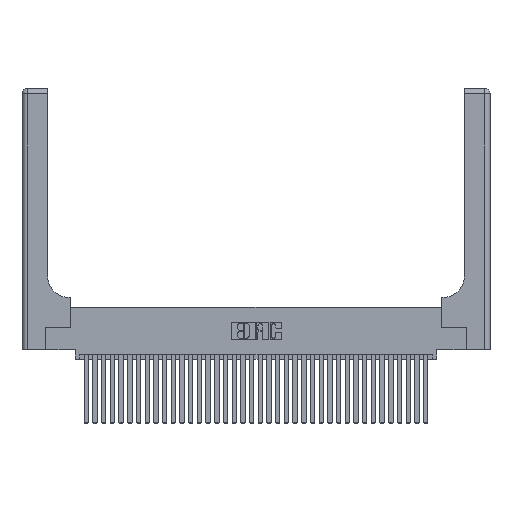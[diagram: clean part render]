
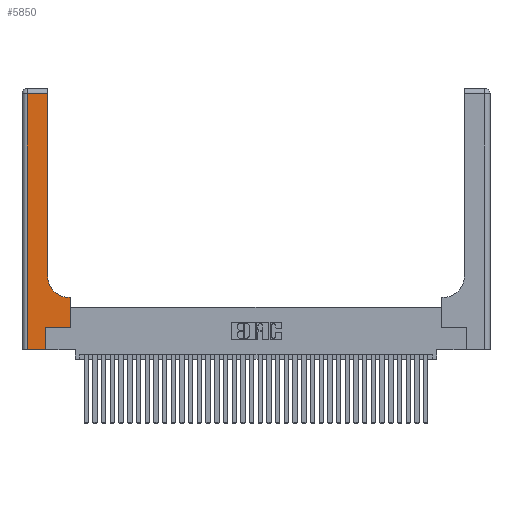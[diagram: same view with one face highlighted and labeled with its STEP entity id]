
A CAD part, top view. The second image highlights one B-rep face of the part: STEP entity #5850.
In plain terms, the highlighted planar face has unit normal (0, 0, 1).
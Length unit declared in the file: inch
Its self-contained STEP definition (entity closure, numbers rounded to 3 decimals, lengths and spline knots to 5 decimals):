
#67 = CARTESIAN_POINT ( 'NONE',  ( 0.5585, 0.25, 0.37 ) ) ;
#528 = CARTESIAN_POINT ( 'NONE',  ( 0.5585, 0.25, 0.37 ) ) ;
#1743 = LINE ( 'NONE', #5448, #31032 ) ;
#1891 = AXIS2_PLACEMENT_3D ( 'NONE', #32146, #15350, #34971 ) ;
#2219 = LINE ( 'NONE', #528, #16575 ) ;
#2608 = ORIENTED_EDGE ( 'NONE', *, *, #20187, .T. ) ;
#3395 = CARTESIAN_POINT ( 'NONE',  ( 0.5585, 0.6, 0.37 ) ) ;
#4171 = VERTEX_POINT ( 'NONE', #67 ) ;
#4239 = VERTEX_POINT ( 'NONE', #3395 ) ;
#5036 = CIRCLE ( 'NONE', #1891, 0.25 ) ;
#5448 = CARTESIAN_POINT ( 'NONE',  ( 0.06, 3., 0.37 ) ) ;
#5617 = EDGE_CURVE ( 'NONE', #33675, #6988, #1743, .T. ) ;
#5850 = ADVANCED_FACE ( 'NONE', ( #25758 ), #29022, .F. ) ;
#6583 = VECTOR ( 'NONE', #8959, 39.37008 ) ;
#6988 = VERTEX_POINT ( 'NONE', #28224 ) ;
#7287 = DIRECTION ( 'NONE',  ( 1., 0., 0. ) ) ;
#8959 = DIRECTION ( 'NONE',  ( 1., 0., 0. ) ) ;
#9021 = DIRECTION ( 'NONE',  ( -1., 0., 0. ) ) ;
#9207 = EDGE_CURVE ( 'NONE', #4239, #23665, #20814, .T. ) ;
#10063 = CARTESIAN_POINT ( 'NONE',  ( 0.2915, 2.94, 0.37 ) ) ;
#11771 = LINE ( 'NONE', #27359, #25807 ) ;
#12192 = AXIS2_PLACEMENT_3D ( 'NONE', #12219, #15021, #34631 ) ;
#12219 = CARTESIAN_POINT ( 'NONE',  ( 0., 3., 0.37 ) ) ;
#13022 = EDGE_CURVE ( 'NONE', #4171, #4239, #2219, .T. ) ;
#13323 = ORIENTED_EDGE ( 'NONE', *, *, #13022, .T. ) ;
#13383 = DIRECTION ( 'NONE',  ( -1., 0., 0. ) ) ;
#14323 = DIRECTION ( 'NONE',  ( 0., 1., 0. ) ) ;
#15021 = DIRECTION ( 'NONE',  ( 0., 0., -1. ) ) ;
#15350 = DIRECTION ( 'NONE',  ( 0., 0., -1. ) ) ;
#16575 = VECTOR ( 'NONE', #17768, 39.37008 ) ;
#17206 = EDGE_CURVE ( 'NONE', #22782, #24727, #25073, .T. ) ;
#17446 = VERTEX_POINT ( 'NONE', #35162 ) ;
#17768 = DIRECTION ( 'NONE',  ( 0., 1., 0. ) ) ;
#17877 = CARTESIAN_POINT ( 'NONE',  ( 0.2915, 0.6, 0.37 ) ) ;
#18522 = CARTESIAN_POINT ( 'NONE',  ( 0.2915, 0.85, 0.37 ) ) ;
#18593 = ORIENTED_EDGE ( 'NONE', *, *, #5617, .T. ) ;
#18896 = EDGE_CURVE ( 'NONE', #24727, #33675, #11771, .T. ) ;
#20073 = ORIENTED_EDGE ( 'NONE', *, *, #18896, .T. ) ;
#20187 = EDGE_CURVE ( 'NONE', #23665, #22782, #5036, .T. ) ;
#20488 = ORIENTED_EDGE ( 'NONE', *, *, #24462, .T. ) ;
#20814 = LINE ( 'NONE', #17877, #28295 ) ;
#21274 = LINE ( 'NONE', #22793, #34390 ) ;
#22116 = DIRECTION ( 'NONE',  ( 0., 1., 0. ) ) ;
#22427 = DIRECTION ( 'NONE',  ( 0., -1., 0. ) ) ;
#22503 = LINE ( 'NONE', #25791, #6583 ) ;
#22567 = VECTOR ( 'NONE', #7287, 39.37008 ) ;
#22782 = VERTEX_POINT ( 'NONE', #18522 ) ;
#22793 = CARTESIAN_POINT ( 'NONE',  ( 0.269, 0., 0.37 ) ) ;
#22799 = EDGE_CURVE ( 'NONE', #33431, #4171, #30030, .T. ) ;
#22839 = EDGE_LOOP ( 'NONE', ( #34150, #20073, #18593, #20488, #26024, #29378, #13323, #36374, #2608 ) ) ;
#23665 = VERTEX_POINT ( 'NONE', #24008 ) ;
#24008 = CARTESIAN_POINT ( 'NONE',  ( 0.5415, 0.6, 0.37 ) ) ;
#24462 = EDGE_CURVE ( 'NONE', #6988, #17446, #22503, .T. ) ;
#24727 = VERTEX_POINT ( 'NONE', #10063 ) ;
#24925 = CARTESIAN_POINT ( 'NONE',  ( 0.2915, 3., 0.37 ) ) ;
#25073 = LINE ( 'NONE', #24925, #30773 ) ;
#25758 = FACE_OUTER_BOUND ( 'NONE', #22839, .T. ) ;
#25791 = CARTESIAN_POINT ( 'NONE',  ( 0., 0., 0.37 ) ) ;
#25807 = VECTOR ( 'NONE', #13383, 39.37008 ) ;
#26024 = ORIENTED_EDGE ( 'NONE', *, *, #34575, .T. ) ;
#26289 = CARTESIAN_POINT ( 'NONE',  ( 0.269, 0.25, 0.37 ) ) ;
#27359 = CARTESIAN_POINT ( 'NONE',  ( 0., 2.94, 0.37 ) ) ;
#28224 = CARTESIAN_POINT ( 'NONE',  ( 0.06, 0., 0.37 ) ) ;
#28295 = VECTOR ( 'NONE', #9021, 39.37008 ) ;
#29022 = PLANE ( 'NONE',  #12192 ) ;
#29378 = ORIENTED_EDGE ( 'NONE', *, *, #22799, .T. ) ;
#29974 = CARTESIAN_POINT ( 'NONE',  ( 0.06, 2.94, 0.37 ) ) ;
#30030 = LINE ( 'NONE', #35313, #22567 ) ;
#30773 = VECTOR ( 'NONE', #22116, 39.37008 ) ;
#31032 = VECTOR ( 'NONE', #22427, 39.37008 ) ;
#32146 = CARTESIAN_POINT ( 'NONE',  ( 0.5415, 0.85, 0.37 ) ) ;
#33431 = VERTEX_POINT ( 'NONE', #26289 ) ;
#33675 = VERTEX_POINT ( 'NONE', #29974 ) ;
#34150 = ORIENTED_EDGE ( 'NONE', *, *, #17206, .T. ) ;
#34390 = VECTOR ( 'NONE', #14323, 39.37008 ) ;
#34575 = EDGE_CURVE ( 'NONE', #17446, #33431, #21274, .T. ) ;
#34631 = DIRECTION ( 'NONE',  ( -1., 0., 0. ) ) ;
#34971 = DIRECTION ( 'NONE',  ( 1., 0., 0. ) ) ;
#35162 = CARTESIAN_POINT ( 'NONE',  ( 0.269, 0., 0.37 ) ) ;
#35313 = CARTESIAN_POINT ( 'NONE',  ( 0.269, 0.25, 0.37 ) ) ;
#36374 = ORIENTED_EDGE ( 'NONE', *, *, #9207, .T. ) ;
